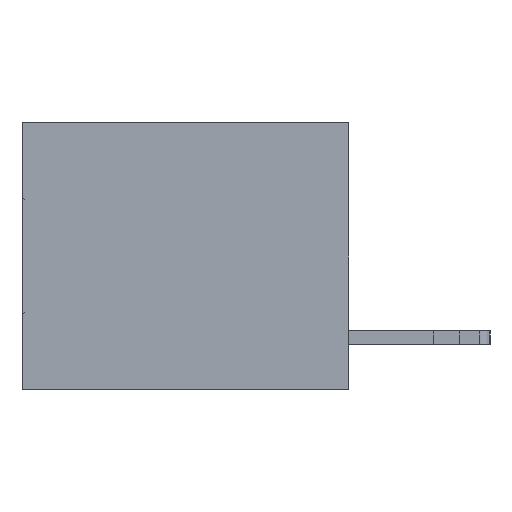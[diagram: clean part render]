
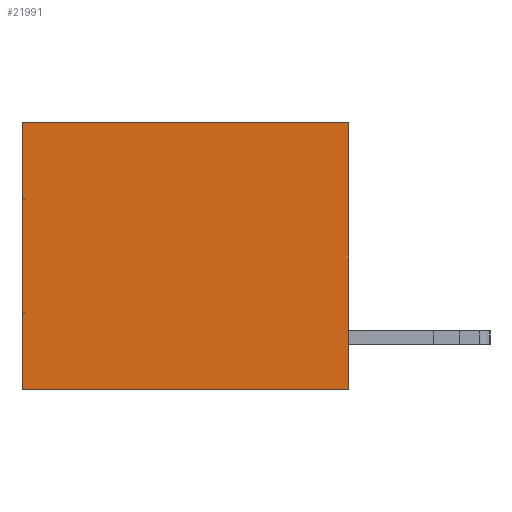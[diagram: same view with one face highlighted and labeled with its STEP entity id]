
A CAD part, left-side view. The second image highlights one B-rep face of the part: STEP entity #21991.
In plain terms, the highlighted planar face has unit normal (-1, 0, 0).
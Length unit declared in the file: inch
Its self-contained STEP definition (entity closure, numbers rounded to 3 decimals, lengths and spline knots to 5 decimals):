
#68 = EDGE_CURVE ( 'NONE', #23036, #25423, #28643, .T. ) ;
#925 = DIRECTION ( 'NONE',  ( 0., 0., -1. ) ) ;
#1035 = EDGE_CURVE ( 'NONE', #25423, #29005, #31462, .T. ) ;
#1403 = EDGE_CURVE ( 'NONE', #23036, #19741, #1850, .T. ) ;
#1547 = EDGE_CURVE ( 'NONE', #19741, #29005, #23954, .T. ) ;
#1850 = LINE ( 'NONE', #25946, #29359 ) ;
#2087 = DIRECTION ( 'NONE',  ( 0., 0., -1. ) ) ;
#2677 = DIRECTION ( 'NONE',  ( 0., 1., 0. ) ) ;
#4832 = VECTOR ( 'NONE', #17308, 39.37008 ) ;
#5376 = EDGE_LOOP ( 'NONE', ( #17416, #19051, #19490, #23125 ) ) ;
#9457 = CARTESIAN_POINT ( 'NONE',  ( 0.3165, 0.6, 0. ) ) ;
#10892 = DIRECTION ( 'NONE',  ( 0., 1., 0. ) ) ;
#11324 = CARTESIAN_POINT ( 'NONE',  ( 0.3165, 0., -0.49 ) ) ;
#12036 = CARTESIAN_POINT ( 'NONE',  ( 0.3165, 0., -0.49 ) ) ;
#12417 = FACE_OUTER_BOUND ( 'NONE', #5376, .T. ) ;
#14954 = CARTESIAN_POINT ( 'NONE',  ( 0.3165, 0., -0.49 ) ) ;
#15581 = CARTESIAN_POINT ( 'NONE',  ( 0.3165, 0., -0.49 ) ) ;
#16505 = CARTESIAN_POINT ( 'NONE',  ( 0.3165, 0., 0. ) ) ;
#17308 = DIRECTION ( 'NONE',  ( 0., 0., -1. ) ) ;
#17416 = ORIENTED_EDGE ( 'NONE', *, *, #1547, .T. ) ;
#17871 = CARTESIAN_POINT ( 'NONE',  ( 0.3165, 0.6, -0.49 ) ) ;
#19051 = ORIENTED_EDGE ( 'NONE', *, *, #1035, .F. ) ;
#19490 = ORIENTED_EDGE ( 'NONE', *, *, #68, .F. ) ;
#19741 = VERTEX_POINT ( 'NONE', #9457 ) ;
#21137 = VECTOR ( 'NONE', #10892, 39.37008 ) ;
#21540 = CARTESIAN_POINT ( 'NONE',  ( 0.3165, 0.6, -0.49 ) ) ;
#21991 = ADVANCED_FACE ( 'NONE', ( #12417 ), #30551, .F. ) ;
#22920 = DIRECTION ( 'NONE',  ( 1., 0., 0. ) ) ;
#23036 = VERTEX_POINT ( 'NONE', #16505 ) ;
#23125 = ORIENTED_EDGE ( 'NONE', *, *, #1403, .T. ) ;
#23954 = LINE ( 'NONE', #21540, #24808 ) ;
#24808 = VECTOR ( 'NONE', #925, 39.37008 ) ;
#25423 = VERTEX_POINT ( 'NONE', #11324 ) ;
#25946 = CARTESIAN_POINT ( 'NONE',  ( 0.3165, 0., 0. ) ) ;
#28643 = LINE ( 'NONE', #12036, #4832 ) ;
#29005 = VERTEX_POINT ( 'NONE', #17871 ) ;
#29359 = VECTOR ( 'NONE', #2677, 39.37008 ) ;
#30551 = PLANE ( 'NONE',  #32180 ) ;
#31462 = LINE ( 'NONE', #15581, #21137 ) ;
#32180 = AXIS2_PLACEMENT_3D ( 'NONE', #14954, #22920, #2087 ) ;
